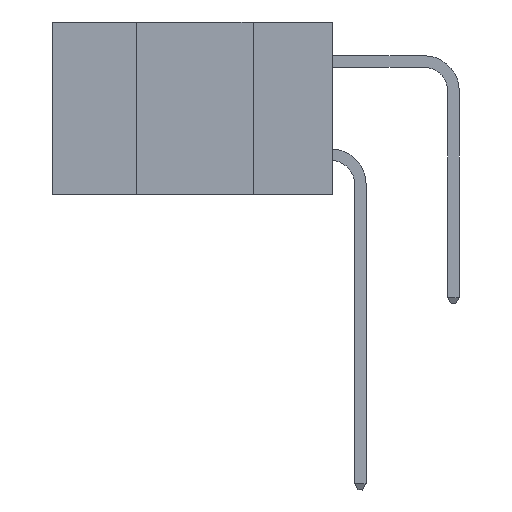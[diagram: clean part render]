
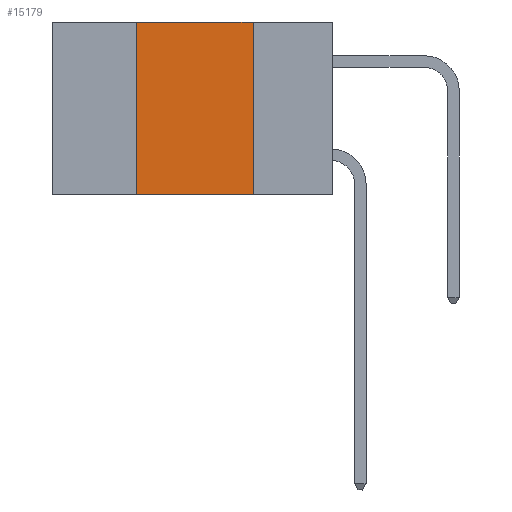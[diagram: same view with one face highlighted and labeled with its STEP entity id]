
A CAD part, left-side view. The second image highlights one B-rep face of the part: STEP entity #15179.
In plain terms, the highlighted planar face has unit normal (-1, 0, 0).
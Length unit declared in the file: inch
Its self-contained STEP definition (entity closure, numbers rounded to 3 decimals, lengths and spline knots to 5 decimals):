
#295 = VECTOR ( 'NONE', #2611, 39.37008 ) ;
#364 = EDGE_LOOP ( 'NONE', ( #1568, #5135, #9916, #1151 ) ) ;
#769 = VERTEX_POINT ( 'NONE', #17619 ) ;
#1080 = CARTESIAN_POINT ( 'NONE',  ( 0., 0.6, -0.37 ) ) ;
#1151 = ORIENTED_EDGE ( 'NONE', *, *, #12624, .T. ) ;
#1171 = DIRECTION ( 'NONE',  ( 0., 0., -1. ) ) ;
#1568 = ORIENTED_EDGE ( 'NONE', *, *, #7155, .F. ) ;
#2191 = LINE ( 'NONE', #18107, #7782 ) ;
#2406 = CARTESIAN_POINT ( 'NONE',  ( 0., 0.17, -0.37 ) ) ;
#2611 = DIRECTION ( 'NONE',  ( 0., -1., 0. ) ) ;
#2843 = VERTEX_POINT ( 'NONE', #2406 ) ;
#3206 = DIRECTION ( 'NONE',  ( 0., -1., 0. ) ) ;
#4219 = CARTESIAN_POINT ( 'NONE',  ( 0., 0.17, -0.37 ) ) ;
#4516 = CARTESIAN_POINT ( 'NONE',  ( 0., 0.42, -0.37 ) ) ;
#5135 = ORIENTED_EDGE ( 'NONE', *, *, #13457, .F. ) ;
#5571 = LINE ( 'NONE', #1080, #295 ) ;
#6526 = CARTESIAN_POINT ( 'NONE',  ( 0., 0.42, 0. ) ) ;
#6543 = VERTEX_POINT ( 'NONE', #4516 ) ;
#7155 = EDGE_CURVE ( 'NONE', #769, #2843, #14138, .T. ) ;
#7672 = VERTEX_POINT ( 'NONE', #6526 ) ;
#7782 = VECTOR ( 'NONE', #3206, 39.37008 ) ;
#8350 = LINE ( 'NONE', #9719, #16046 ) ;
#9719 = CARTESIAN_POINT ( 'NONE',  ( 0., 0.42, -0.37 ) ) ;
#9916 = ORIENTED_EDGE ( 'NONE', *, *, #17515, .F. ) ;
#11324 = FACE_OUTER_BOUND ( 'NONE', #364, .T. ) ;
#11416 = CARTESIAN_POINT ( 'NONE',  ( 0., 0.6, 0. ) ) ;
#12624 = EDGE_CURVE ( 'NONE', #6543, #2843, #5571, .T. ) ;
#13457 = EDGE_CURVE ( 'NONE', #7672, #769, #2191, .T. ) ;
#13615 = AXIS2_PLACEMENT_3D ( 'NONE', #11416, #15927, #14102 ) ;
#14102 = DIRECTION ( 'NONE',  ( 0., 0., -1. ) ) ;
#14138 = LINE ( 'NONE', #4219, #15259 ) ;
#15179 = ADVANCED_FACE ( 'NONE', ( #11324 ), #18771, .F. ) ;
#15259 = VECTOR ( 'NONE', #1171, 39.37008 ) ;
#15560 = DIRECTION ( 'NONE',  ( 0., 0., 1. ) ) ;
#15927 = DIRECTION ( 'NONE',  ( 1., 0., 0. ) ) ;
#16046 = VECTOR ( 'NONE', #15560, 39.37008 ) ;
#17515 = EDGE_CURVE ( 'NONE', #6543, #7672, #8350, .T. ) ;
#17619 = CARTESIAN_POINT ( 'NONE',  ( 0., 0.17, 0. ) ) ;
#18107 = CARTESIAN_POINT ( 'NONE',  ( 0., 0.6, 0. ) ) ;
#18771 = PLANE ( 'NONE',  #13615 ) ;
